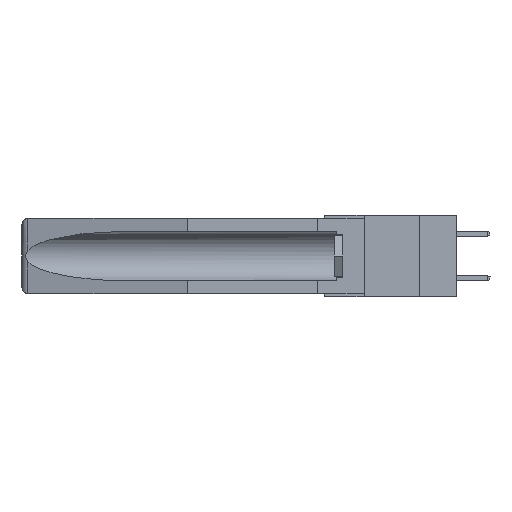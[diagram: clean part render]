
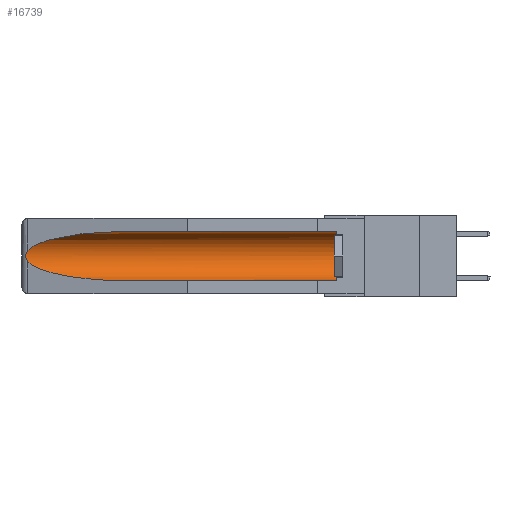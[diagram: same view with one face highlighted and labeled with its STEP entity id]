
A CAD part, left-side view. The second image highlights one B-rep face of the part: STEP entity #16739.
In plain terms, the highlighted cylindrical face has radius 2.857 mm (diameter 5.715 mm), a partial arc.
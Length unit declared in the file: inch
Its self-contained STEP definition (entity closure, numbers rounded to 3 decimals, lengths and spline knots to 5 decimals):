
#156 = LINE ( 'NONE', #22640, #23233 ) ;
#773 = CARTESIAN_POINT ( 'NONE',  ( 0.155, 0.126, -0.284 ) ) ;
#1009 = CARTESIAN_POINT ( 'NONE',  ( 0.25451, 1.48313, -0.24835 ) ) ;
#1651 = VERTEX_POINT ( 'NONE', #12388 ) ;
#1820 = CARTESIAN_POINT ( 'NONE',  ( 0.25451, 1.48313, -0.09465 ) ) ;
#2398 = CARTESIAN_POINT ( 'NONE',  ( 0.155, -0.30754, -0.1715 ) ) ;
#2575 = DIRECTION ( 'NONE',  ( 0., 0., 1. ) ) ;
#2780 = CARTESIAN_POINT ( 'NONE',  ( 0.155, 1.07973, -0.059 ) ) ;
#2847 = EDGE_CURVE ( 'NONE', #5063, #1651, #3971, .T. ) ;
#3123 = CARTESIAN_POINT ( 'NONE',  ( 0.26654, 1.53092, -0.15636 ) ) ;
#3209 = CARTESIAN_POINT ( 'NONE',  ( 0.2675, 1.53308, -0.16763 ) ) ;
#3355 = CARTESIAN_POINT ( 'NONE',  ( 0.21114, 1.30732, -0.284 ) ) ;
#3382 = EDGE_CURVE ( 'NONE', #18727, #11658, #19037, .T. ) ;
#3437 = ORIENTED_EDGE ( 'NONE', *, *, #3382, .T. ) ;
#3963 = DIRECTION ( 'NONE',  ( 0., 0., 1. ) ) ;
#3971 = CIRCLE ( 'NONE', #13305, 0.1125 ) ;
#4498 = EDGE_CURVE ( 'NONE', #5063, #11658, #156, .T. ) ;
#4892 = CARTESIAN_POINT ( 'NONE',  ( 0.26537, 1.52718, -0.19328 ) ) ;
#4984 = CARTESIAN_POINT ( 'NONE',  ( 0.155, 1.07973, -0.284 ) ) ;
#5063 = VERTEX_POINT ( 'NONE', #773 ) ;
#5408 = CARTESIAN_POINT ( 'NONE',  ( 0.26537, 1.52718, -0.19328 ) ) ;
#5632 = B_SPLINE_CURVE_WITH_KNOTS ( 'NONE', 3,
 ( #18328, #15999, #3123, #27017, #3209, #7624, #18423, #13899, #26645, #5408 ),
 .UNSPECIFIED., .F., .F.,
 ( 4, 2, 2, 2, 4 ),
 ( 0., 0.00029, 0.00058, 0.00087, 0.00117 ),
 .UNSPECIFIED. ) ;
#6863 = EDGE_LOOP ( 'NONE', ( #28043, #9433, #3437, #9574, #13179, #9626 ) ) ;
#7263 = FACE_OUTER_BOUND ( 'NONE', #6863, .T. ) ;
#7624 = CARTESIAN_POINT ( 'NONE',  ( 0.2675, 1.53308, -0.17534 ) ) ;
#7765 = DIRECTION ( 'NONE',  ( 0., 1., 0. ) ) ;
#8952 = CYLINDRICAL_SURFACE ( 'NONE', #25297, 0.1125 ) ;
#9433 = ORIENTED_EDGE ( 'NONE', *, *, #22253, .T. ) ;
#9574 = ORIENTED_EDGE ( 'NONE', *, *, #4498, .F. ) ;
#9626 = ORIENTED_EDGE ( 'NONE', *, *, #12362, .T. ) ;
#10593 = CARTESIAN_POINT ( 'NONE',  ( 0.155, 1.07973, -0.059 ) ) ;
#11658 = VERTEX_POINT ( 'NONE', #4984 ) ;
#12362 = EDGE_CURVE ( 'NONE', #1651, #27327, #22458, .T. ) ;
#12388 = CARTESIAN_POINT ( 'NONE',  ( 0.155, 0.126, -0.059 ) ) ;
#12844 = DIRECTION ( 'NONE',  ( 0., 1., 0. ) ) ;
#13179 = ORIENTED_EDGE ( 'NONE', *, *, #2847, .T. ) ;
#13305 = AXIS2_PLACEMENT_3D ( 'NONE', #14746, #21068, #3963 ) ;
#13423 = DIRECTION ( 'NONE',  ( 0., 1., 0. ) ) ;
#13899 = CARTESIAN_POINT ( 'NONE',  ( 0.26655, 1.53094, -0.18657 ) ) ;
#14746 = CARTESIAN_POINT ( 'NONE',  ( 0.155, 0.126, -0.1715 ) ) ;
#15999 = CARTESIAN_POINT ( 'NONE',  ( 0.26597, 1.52961, -0.15275 ) ) ;
#16301 = CARTESIAN_POINT ( 'NONE',  ( 0.26537, 1.52718, -0.14972 ) ) ;
#16315 = CARTESIAN_POINT ( 'NONE',  ( 0.155, 1.07973, -0.284 ) ) ;
#16739 = ADVANCED_FACE ( 'NONE', ( #7263 ), #8952, .F. ) ;
#18328 = CARTESIAN_POINT ( 'NONE',  ( 0.26537, 1.52718, -0.14972 ) ) ;
#18354 = VECTOR ( 'NONE', #12844, 39.37008 ) ;
#18423 = CARTESIAN_POINT ( 'NONE',  ( 0.2673, 1.53269, -0.17917 ) ) ;
#18727 = VERTEX_POINT ( 'NONE', #4892 ) ;
#18901 = EDGE_CURVE ( 'NONE', #27327, #23042, #25791, .T. ) ;
#19037 =( BOUNDED_CURVE ( )  B_SPLINE_CURVE ( 3, ( #27159, #1009, #3355, #16315 ),
 .UNSPECIFIED., .F., .F. ) 
 B_SPLINE_CURVE_WITH_KNOTS ( ( 4, 4 ),
 ( 0.1948, 1.5708 ),
 .UNSPECIFIED. ) 
 CURVE ( )  GEOMETRIC_REPRESENTATION_ITEM ( )  RATIONAL_B_SPLINE_CURVE ( ( 1., 0.848, 0.848, 1. ) ) 
 REPRESENTATION_ITEM ( '' )  );
#19288 = CARTESIAN_POINT ( 'NONE',  ( 0.155, -0.30754, -0.059 ) ) ;
#21068 = DIRECTION ( 'NONE',  ( 0., -1., 0. ) ) ;
#22253 = EDGE_CURVE ( 'NONE', #23042, #18727, #5632, .T. ) ;
#22458 = LINE ( 'NONE', #19288, #18354 ) ;
#22640 = CARTESIAN_POINT ( 'NONE',  ( 0.155, -0.30754, -0.284 ) ) ;
#23042 = VERTEX_POINT ( 'NONE', #16301 ) ;
#23233 = VECTOR ( 'NONE', #7765, 39.37008 ) ;
#25297 = AXIS2_PLACEMENT_3D ( 'NONE', #2398, #13423, #2575 ) ;
#25791 =( BOUNDED_CURVE ( )  B_SPLINE_CURVE ( 3, ( #10593, #27618, #1820, #27897 ),
 .UNSPECIFIED., .F., .F. ) 
 B_SPLINE_CURVE_WITH_KNOTS ( ( 4, 4 ),
 ( 4.71239, 6.08839 ),
 .UNSPECIFIED. ) 
 CURVE ( )  GEOMETRIC_REPRESENTATION_ITEM ( )  RATIONAL_B_SPLINE_CURVE ( ( 1., 0.848, 0.848, 1. ) ) 
 REPRESENTATION_ITEM ( '' )  );
#26645 = CARTESIAN_POINT ( 'NONE',  ( 0.26597, 1.5296, -0.19026 ) ) ;
#27017 = CARTESIAN_POINT ( 'NONE',  ( 0.2673, 1.5327, -0.16383 ) ) ;
#27159 = CARTESIAN_POINT ( 'NONE',  ( 0.26537, 1.52718, -0.19328 ) ) ;
#27327 = VERTEX_POINT ( 'NONE', #2780 ) ;
#27618 = CARTESIAN_POINT ( 'NONE',  ( 0.21114, 1.30732, -0.059 ) ) ;
#27897 = CARTESIAN_POINT ( 'NONE',  ( 0.26537, 1.52718, -0.14972 ) ) ;
#28043 = ORIENTED_EDGE ( 'NONE', *, *, #18901, .T. ) ;
